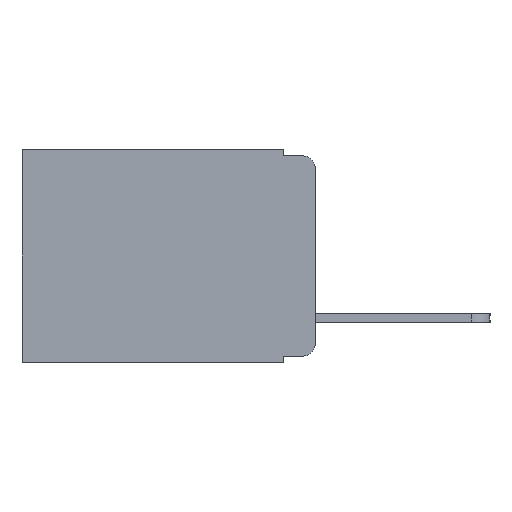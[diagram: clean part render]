
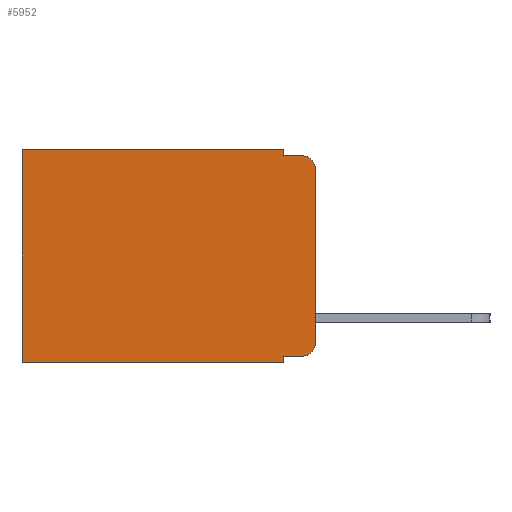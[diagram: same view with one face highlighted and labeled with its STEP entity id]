
A CAD part, left-side view. The second image highlights one B-rep face of the part: STEP entity #5952.
In plain terms, the highlighted planar face has unit normal (-1, 0, 0).
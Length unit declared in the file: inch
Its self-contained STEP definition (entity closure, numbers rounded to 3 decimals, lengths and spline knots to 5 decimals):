
#25 = VECTOR ( 'NONE', #2316, 39.37008 ) ;
#284 = VECTOR ( 'NONE', #5734, 39.37008 ) ;
#1294 = CARTESIAN_POINT ( 'NONE',  ( 0.298, 0.051, -0.01 ) ) ;
#1799 = VECTOR ( 'NONE', #5997, 39.37008 ) ;
#2316 = DIRECTION ( 'NONE',  ( 0., 0., -1. ) ) ;
#3178 = VERTEX_POINT ( 'NONE', #13975 ) ;
#3206 = DIRECTION ( 'NONE',  ( -1., 0., 0. ) ) ;
#3281 = CARTESIAN_POINT ( 'NONE',  ( 0.298, 0., -0.313 ) ) ;
#3384 = VERTEX_POINT ( 'NONE', #22526 ) ;
#3559 = VERTEX_POINT ( 'NONE', #1294 ) ;
#3998 = DIRECTION ( 'NONE',  ( 0., -1., 0. ) ) ;
#4746 = DIRECTION ( 'NONE',  ( 0., 1., 0. ) ) ;
#5190 = EDGE_CURVE ( 'NONE', #13585, #3559, #22863, .T. ) ;
#5475 = CIRCLE ( 'NONE', #18872, 0.02 ) ;
#5726 = EDGE_CURVE ( 'NONE', #19518, #8787, #5475, .T. ) ;
#5734 = DIRECTION ( 'NONE',  ( 0., 0., -1. ) ) ;
#5952 = ADVANCED_FACE ( 'NONE', ( #15167 ), #22839, .F. ) ;
#5997 = DIRECTION ( 'NONE',  ( 0., -1., 0. ) ) ;
#6178 = AXIS2_PLACEMENT_3D ( 'NONE', #22761, #7046, #9664 ) ;
#6444 = CARTESIAN_POINT ( 'NONE',  ( 0.298, 0.051, 0. ) ) ;
#6687 = CARTESIAN_POINT ( 'NONE',  ( 0.298, 0.473, -0.343 ) ) ;
#6939 = EDGE_CURVE ( 'NONE', #3178, #19518, #11378, .T. ) ;
#6944 = CARTESIAN_POINT ( 'NONE',  ( 0.298, 0., -0.343 ) ) ;
#7046 = DIRECTION ( 'NONE',  ( 1., 0., 0. ) ) ;
#7104 = DIRECTION ( 'NONE',  ( 0., 0., -1. ) ) ;
#7404 = ORIENTED_EDGE ( 'NONE', *, *, #18439, .T. ) ;
#7409 = DIRECTION ( 'NONE',  ( 0., 0., -1. ) ) ;
#8090 = DIRECTION ( 'NONE',  ( 0., 0., -1. ) ) ;
#8159 = EDGE_CURVE ( 'NONE', #3178, #18488, #21126, .T. ) ;
#8254 = VECTOR ( 'NONE', #7104, 39.37008 ) ;
#8787 = VERTEX_POINT ( 'NONE', #3281 ) ;
#9616 = LINE ( 'NONE', #12982, #25 ) ;
#9664 = DIRECTION ( 'NONE',  ( 0., 0., -1. ) ) ;
#9932 = AXIS2_PLACEMENT_3D ( 'NONE', #13836, #3206, #15565 ) ;
#9936 = ORIENTED_EDGE ( 'NONE', *, *, #5726, .T. ) ;
#9982 = LINE ( 'NONE', #13593, #22316 ) ;
#10576 = CARTESIAN_POINT ( 'NONE',  ( 0.298, 0., -0.03 ) ) ;
#11378 = LINE ( 'NONE', #14593, #20086 ) ;
#11611 = VERTEX_POINT ( 'NONE', #10576 ) ;
#12052 = EDGE_CURVE ( 'NONE', #11611, #8787, #9616, .T. ) ;
#12982 = CARTESIAN_POINT ( 'NONE',  ( 0.298, 0., 0. ) ) ;
#13237 = EDGE_CURVE ( 'NONE', #3559, #19669, #20591, .T. ) ;
#13585 = VERTEX_POINT ( 'NONE', #15284 ) ;
#13593 = CARTESIAN_POINT ( 'NONE',  ( 0.298, 0., 0. ) ) ;
#13836 = CARTESIAN_POINT ( 'NONE',  ( 0.298, 0.02, -0.03 ) ) ;
#13975 = CARTESIAN_POINT ( 'NONE',  ( 0.298, 0.051, -0.333 ) ) ;
#14047 = CARTESIAN_POINT ( 'NONE',  ( 0.298, 0.02, -0.333 ) ) ;
#14146 = LINE ( 'NONE', #6944, #18789 ) ;
#14379 = EDGE_CURVE ( 'NONE', #3384, #19428, #18097, .T. ) ;
#14593 = CARTESIAN_POINT ( 'NONE',  ( 0.298, 0.051, -0.333 ) ) ;
#14831 = CARTESIAN_POINT ( 'NONE',  ( 0.298, 0.051, -0.01 ) ) ;
#15167 = FACE_OUTER_BOUND ( 'NONE', #22156, .T. ) ;
#15284 = CARTESIAN_POINT ( 'NONE',  ( 0.298, 0.051, 0. ) ) ;
#15565 = DIRECTION ( 'NONE',  ( 0., 0., -1. ) ) ;
#15678 = ORIENTED_EDGE ( 'NONE', *, *, #6939, .T. ) ;
#16326 = CARTESIAN_POINT ( 'NONE',  ( 0.298, 0.473, 0. ) ) ;
#16698 = ORIENTED_EDGE ( 'NONE', *, *, #17894, .T. ) ;
#17894 = EDGE_CURVE ( 'NONE', #11611, #19669, #19871, .T. ) ;
#17965 = EDGE_CURVE ( 'NONE', #18488, #19428, #14146, .T. ) ;
#18097 = LINE ( 'NONE', #16326, #284 ) ;
#18439 = EDGE_CURVE ( 'NONE', #13585, #3384, #9982, .T. ) ;
#18488 = VERTEX_POINT ( 'NONE', #22367 ) ;
#18650 = ORIENTED_EDGE ( 'NONE', *, *, #8159, .F. ) ;
#18789 = VECTOR ( 'NONE', #19225, 39.37008 ) ;
#18872 = AXIS2_PLACEMENT_3D ( 'NONE', #22943, #22913, #8090 ) ;
#19225 = DIRECTION ( 'NONE',  ( 0., 1., 0. ) ) ;
#19352 = ORIENTED_EDGE ( 'NONE', *, *, #13237, .F. ) ;
#19428 = VERTEX_POINT ( 'NONE', #6687 ) ;
#19518 = VERTEX_POINT ( 'NONE', #14047 ) ;
#19669 = VERTEX_POINT ( 'NONE', #21432 ) ;
#19720 = ORIENTED_EDGE ( 'NONE', *, *, #17965, .F. ) ;
#19745 = ORIENTED_EDGE ( 'NONE', *, *, #5190, .F. ) ;
#19871 = CIRCLE ( 'NONE', #9932, 0.02 ) ;
#20086 = VECTOR ( 'NONE', #3998, 39.37008 ) ;
#20282 = ORIENTED_EDGE ( 'NONE', *, *, #12052, .F. ) ;
#20582 = ORIENTED_EDGE ( 'NONE', *, *, #14379, .T. ) ;
#20591 = LINE ( 'NONE', #14831, #1799 ) ;
#21126 = LINE ( 'NONE', #22921, #8254 ) ;
#21432 = CARTESIAN_POINT ( 'NONE',  ( 0.298, 0.02, -0.01 ) ) ;
#22156 = EDGE_LOOP ( 'NONE', ( #20282, #16698, #19352, #19745, #7404, #20582, #19720, #18650, #15678, #9936 ) ) ;
#22311 = VECTOR ( 'NONE', #7409, 39.37008 ) ;
#22316 = VECTOR ( 'NONE', #4746, 39.37008 ) ;
#22367 = CARTESIAN_POINT ( 'NONE',  ( 0.298, 0.051, -0.343 ) ) ;
#22526 = CARTESIAN_POINT ( 'NONE',  ( 0.298, 0.473, 0. ) ) ;
#22761 = CARTESIAN_POINT ( 'NONE',  ( 0.298, 0., 0. ) ) ;
#22839 = PLANE ( 'NONE',  #6178 ) ;
#22863 = LINE ( 'NONE', #6444, #22311 ) ;
#22913 = DIRECTION ( 'NONE',  ( -1., 0., 0. ) ) ;
#22921 = CARTESIAN_POINT ( 'NONE',  ( 0.298, 0.051, 0. ) ) ;
#22943 = CARTESIAN_POINT ( 'NONE',  ( 0.298, 0.02, -0.313 ) ) ;
